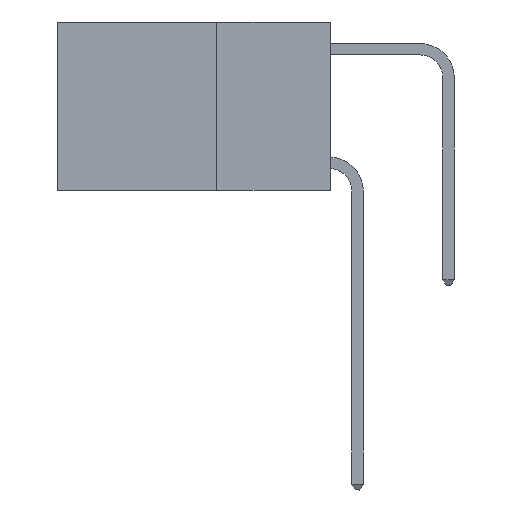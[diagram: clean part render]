
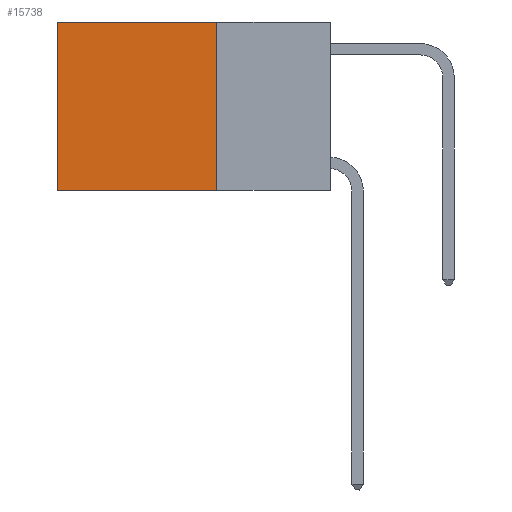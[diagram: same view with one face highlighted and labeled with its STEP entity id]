
A CAD part, left-side view. The second image highlights one B-rep face of the part: STEP entity #15738.
In plain terms, the highlighted planar face has unit normal (-1, 0, 0).
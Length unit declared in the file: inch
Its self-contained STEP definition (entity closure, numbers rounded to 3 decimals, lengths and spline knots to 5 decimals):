
#221 = VECTOR ( 'NONE', #3387, 39.37008 ) ;
#713 = LINE ( 'NONE', #21401, #19373 ) ;
#1249 = EDGE_CURVE ( 'NONE', #22100, #16328, #4598, .T. ) ;
#1504 = VERTEX_POINT ( 'NONE', #13426 ) ;
#1657 = DIRECTION ( 'NONE',  ( 0., 1., 0. ) ) ;
#2685 = ORIENTED_EDGE ( 'NONE', *, *, #10004, .T. ) ;
#3387 = DIRECTION ( 'NONE',  ( 0., 0., -1. ) ) ;
#4598 = LINE ( 'NONE', #17147, #221 ) ;
#5816 = CARTESIAN_POINT ( 'NONE',  ( 0.2625, 0.25, 0. ) ) ;
#6981 = VECTOR ( 'NONE', #1657, 39.37008 ) ;
#8305 = CARTESIAN_POINT ( 'NONE',  ( 0.2625, 0.25, 0. ) ) ;
#9078 = AXIS2_PLACEMENT_3D ( 'NONE', #8305, #10697, #29078 ) ;
#10004 = EDGE_CURVE ( 'NONE', #22100, #14338, #25566, .T. ) ;
#10697 = DIRECTION ( 'NONE',  ( 1., 0., 0. ) ) ;
#12370 = DIRECTION ( 'NONE',  ( 0., 0., -1. ) ) ;
#13237 = ORIENTED_EDGE ( 'NONE', *, *, #15549, .T. ) ;
#13426 = CARTESIAN_POINT ( 'NONE',  ( 0.2625, 0.6, -0.37 ) ) ;
#13591 = EDGE_CURVE ( 'NONE', #16328, #1504, #22426, .T. ) ;
#14338 = VERTEX_POINT ( 'NONE', #24480 ) ;
#15549 = EDGE_CURVE ( 'NONE', #14338, #1504, #713, .T. ) ;
#15738 = ADVANCED_FACE ( 'NONE', ( #28764 ), #24249, .F. ) ;
#16328 = VERTEX_POINT ( 'NONE', #26803 ) ;
#17147 = CARTESIAN_POINT ( 'NONE',  ( 0.2625, 0.25, 0. ) ) ;
#19373 = VECTOR ( 'NONE', #12370, 39.37008 ) ;
#19792 = CARTESIAN_POINT ( 'NONE',  ( 0.2625, 0.25, -0.37 ) ) ;
#20005 = EDGE_LOOP ( 'NONE', ( #13237, #23006, #22464, #2685 ) ) ;
#21401 = CARTESIAN_POINT ( 'NONE',  ( 0.2625, 0.6, 0. ) ) ;
#21893 = DIRECTION ( 'NONE',  ( 0., 1., 0. ) ) ;
#22100 = VERTEX_POINT ( 'NONE', #26764 ) ;
#22426 = LINE ( 'NONE', #19792, #6981 ) ;
#22464 = ORIENTED_EDGE ( 'NONE', *, *, #1249, .F. ) ;
#23006 = ORIENTED_EDGE ( 'NONE', *, *, #13591, .F. ) ;
#24249 = PLANE ( 'NONE',  #9078 ) ;
#24480 = CARTESIAN_POINT ( 'NONE',  ( 0.2625, 0.6, 0. ) ) ;
#25566 = LINE ( 'NONE', #5816, #26652 ) ;
#26652 = VECTOR ( 'NONE', #21893, 39.37008 ) ;
#26764 = CARTESIAN_POINT ( 'NONE',  ( 0.2625, 0.25, 0. ) ) ;
#26803 = CARTESIAN_POINT ( 'NONE',  ( 0.2625, 0.25, -0.37 ) ) ;
#28764 = FACE_OUTER_BOUND ( 'NONE', #20005, .T. ) ;
#29078 = DIRECTION ( 'NONE',  ( 0., 0., -1. ) ) ;
